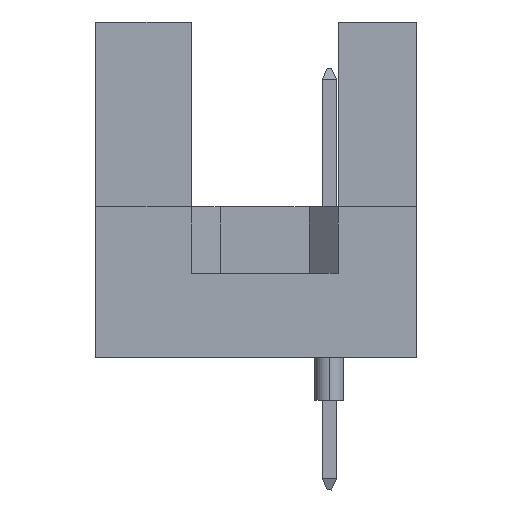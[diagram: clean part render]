
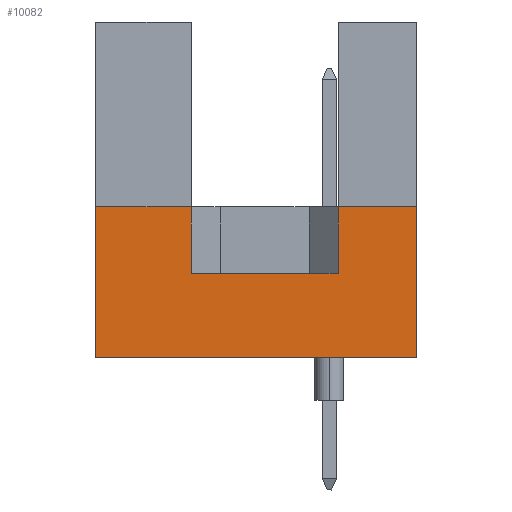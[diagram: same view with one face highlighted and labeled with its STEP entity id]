
A CAD part, left-side view. The second image highlights one B-rep face of the part: STEP entity #10082.
In plain terms, the highlighted planar face has unit normal (-1, 0, 0).
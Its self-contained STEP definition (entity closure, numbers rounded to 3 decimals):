
#1480 = EDGE_CURVE ( 'NONE', #7184, #13312, #13981, .T. ) ;
#1541 = CARTESIAN_POINT ( 'NONE',  ( -47.5, 11.1, 0. ) ) ;
#1717 = DIRECTION ( 'NONE',  ( 0., -1., 0. ) ) ;
#1801 = CARTESIAN_POINT ( 'NONE',  ( -47.5, 11.1, 5.2 ) ) ;
#2027 = DIRECTION ( 'NONE',  ( 1., 0., 0. ) ) ;
#2050 = CARTESIAN_POINT ( 'NONE',  ( -47.5, 0., 0. ) ) ;
#2481 = VERTEX_POINT ( 'NONE', #8881 ) ;
#2739 = EDGE_CURVE ( 'NONE', #10321, #2481, #3796, .T. ) ;
#2932 = LINE ( 'NONE', #14313, #3308 ) ;
#3308 = VECTOR ( 'NONE', #5349, 1000. ) ;
#3371 = VECTOR ( 'NONE', #11953, 1000. ) ;
#3393 = ORIENTED_EDGE ( 'NONE', *, *, #1480, .F. ) ;
#3796 = LINE ( 'NONE', #14708, #10715 ) ;
#4170 = VERTEX_POINT ( 'NONE', #6249 ) ;
#4246 = EDGE_CURVE ( 'NONE', #2481, #7184, #2932, .T. ) ;
#5133 = ORIENTED_EDGE ( 'NONE', *, *, #15569, .T. ) ;
#5250 = VECTOR ( 'NONE', #6322, 1000. ) ;
#5328 = CARTESIAN_POINT ( 'NONE',  ( -47.5, 11.1, 0. ) ) ;
#5349 = DIRECTION ( 'NONE',  ( 0., 0., 1. ) ) ;
#5379 = DIRECTION ( 'NONE',  ( 0., 0., 1. ) ) ;
#5505 = DIRECTION ( 'NONE',  ( 0., 0., -1. ) ) ;
#5891 = ORIENTED_EDGE ( 'NONE', *, *, #4246, .F. ) ;
#6078 = AXIS2_PLACEMENT_3D ( 'NONE', #9334, #2027, #5505 ) ;
#6143 = DIRECTION ( 'NONE',  ( 0., -1., 0. ) ) ;
#6249 = CARTESIAN_POINT ( 'NONE',  ( -47.5, 7.79, 5.2 ) ) ;
#6322 = DIRECTION ( 'NONE',  ( 0., -1., 0. ) ) ;
#6559 = DIRECTION ( 'NONE',  ( 0., -1., 0. ) ) ;
#6886 = ORIENTED_EDGE ( 'NONE', *, *, #14649, .T. ) ;
#6921 = CARTESIAN_POINT ( 'NONE',  ( -47.5, 7.79, 2.9 ) ) ;
#7184 = VERTEX_POINT ( 'NONE', #8121 ) ;
#7204 = ORIENTED_EDGE ( 'NONE', *, *, #14942, .F. ) ;
#7434 = VERTEX_POINT ( 'NONE', #5328 ) ;
#7878 = CARTESIAN_POINT ( 'NONE',  ( -47.5, 11.1, 5.2 ) ) ;
#8121 = CARTESIAN_POINT ( 'NONE',  ( -47.5, 2.71, 5.2 ) ) ;
#8881 = CARTESIAN_POINT ( 'NONE',  ( -47.5, 2.71, 2.9 ) ) ;
#9173 = PLANE ( 'NONE',  #6078 ) ;
#9321 = VECTOR ( 'NONE', #14679, 1000. ) ;
#9334 = CARTESIAN_POINT ( 'NONE',  ( -47.5, 11.1, 0. ) ) ;
#9614 = VERTEX_POINT ( 'NONE', #9861 ) ;
#9861 = CARTESIAN_POINT ( 'NONE',  ( -47.5, 0., 0. ) ) ;
#10082 = ADVANCED_FACE ( 'NONE', ( #11768 ), #9173, .F. ) ;
#10321 = VERTEX_POINT ( 'NONE', #6921 ) ;
#10715 = VECTOR ( 'NONE', #6143, 1000. ) ;
#10859 = ORIENTED_EDGE ( 'NONE', *, *, #2739, .F. ) ;
#11462 = CARTESIAN_POINT ( 'NONE',  ( -47.5, 0., 5.2 ) ) ;
#11768 = FACE_OUTER_BOUND ( 'NONE', #15416, .T. ) ;
#11953 = DIRECTION ( 'NONE',  ( 0., 0., 1. ) ) ;
#12993 = ORIENTED_EDGE ( 'NONE', *, *, #13680, .T. ) ;
#13222 = VECTOR ( 'NONE', #5379, 1000. ) ;
#13259 = LINE ( 'NONE', #2050, #3371 ) ;
#13294 = EDGE_CURVE ( 'NONE', #13951, #4170, #14159, .T. ) ;
#13312 = VERTEX_POINT ( 'NONE', #11462 ) ;
#13470 = CARTESIAN_POINT ( 'NONE',  ( -47.5, 11.1, 5.2 ) ) ;
#13538 = CARTESIAN_POINT ( 'NONE',  ( -47.5, 7.79, 2.9 ) ) ;
#13680 = EDGE_CURVE ( 'NONE', #7434, #9614, #14060, .T. ) ;
#13951 = VERTEX_POINT ( 'NONE', #13470 ) ;
#13981 = LINE ( 'NONE', #7878, #5250 ) ;
#14060 = LINE ( 'NONE', #1541, #15026 ) ;
#14159 = LINE ( 'NONE', #1801, #15268 ) ;
#14313 = CARTESIAN_POINT ( 'NONE',  ( -47.5, 2.71, 2.9 ) ) ;
#14339 = LINE ( 'NONE', #15318, #13222 ) ;
#14649 = EDGE_CURVE ( 'NONE', #10321, #4170, #15975, .T. ) ;
#14679 = DIRECTION ( 'NONE',  ( 0., 0., 1. ) ) ;
#14708 = CARTESIAN_POINT ( 'NONE',  ( -47.5, 7.79, 2.9 ) ) ;
#14942 = EDGE_CURVE ( 'NONE', #7434, #13951, #14339, .T. ) ;
#15026 = VECTOR ( 'NONE', #6559, 1000. ) ;
#15268 = VECTOR ( 'NONE', #1717, 1000. ) ;
#15318 = CARTESIAN_POINT ( 'NONE',  ( -47.5, 11.1, 0. ) ) ;
#15416 = EDGE_LOOP ( 'NONE', ( #10859, #6886, #15518, #7204, #12993, #5133, #3393, #5891 ) ) ;
#15518 = ORIENTED_EDGE ( 'NONE', *, *, #13294, .F. ) ;
#15569 = EDGE_CURVE ( 'NONE', #9614, #13312, #13259, .T. ) ;
#15975 = LINE ( 'NONE', #13538, #9321 ) ;
